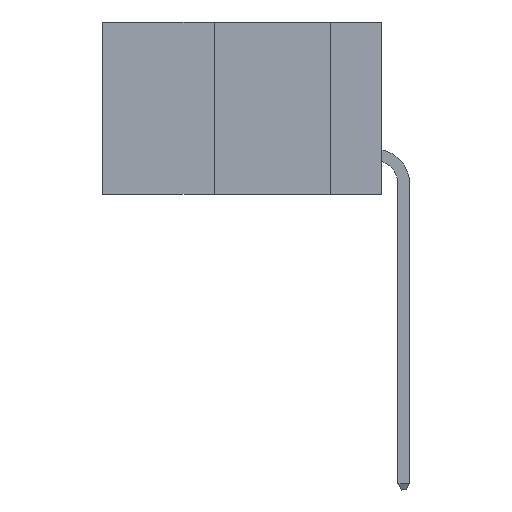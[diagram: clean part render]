
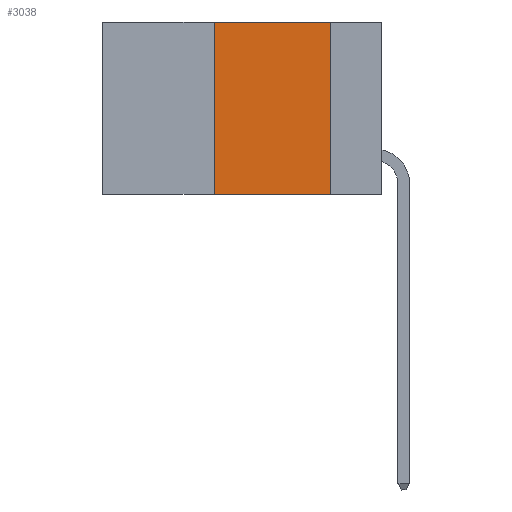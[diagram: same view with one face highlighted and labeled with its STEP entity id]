
A CAD part, left-side view. The second image highlights one B-rep face of the part: STEP entity #3038.
In plain terms, the highlighted planar face has unit normal (-1, 0, 0).
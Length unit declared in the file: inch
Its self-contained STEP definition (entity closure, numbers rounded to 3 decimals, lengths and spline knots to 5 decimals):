
#28 = CARTESIAN_POINT ( 'NONE',  ( 0., 0.36, -0.37 ) ) ;
#169 = DIRECTION ( 'NONE',  ( 0., -1., 0. ) ) ;
#285 = ORIENTED_EDGE ( 'NONE', *, *, #8135, .F. ) ;
#476 = VERTEX_POINT ( 'NONE', #6711 ) ;
#570 = DIRECTION ( 'NONE',  ( 1., 0., 0. ) ) ;
#1291 = ORIENTED_EDGE ( 'NONE', *, *, #11088, .F. ) ;
#1450 = EDGE_LOOP ( 'NONE', ( #8328, #1291, #285, #11662 ) ) ;
#1872 = LINE ( 'NONE', #11894, #10396 ) ;
#3038 = ADVANCED_FACE ( 'NONE', ( #11438 ), #11266, .F. ) ;
#4275 = VERTEX_POINT ( 'NONE', #7048 ) ;
#5135 = VERTEX_POINT ( 'NONE', #7975 ) ;
#5703 = CARTESIAN_POINT ( 'NONE',  ( 0., 0.6, 0. ) ) ;
#5816 = CARTESIAN_POINT ( 'NONE',  ( 0., 0.11, 0. ) ) ;
#6197 = LINE ( 'NONE', #13666, #11407 ) ;
#6268 = VECTOR ( 'NONE', #13114, 39.37008 ) ;
#6703 = DIRECTION ( 'NONE',  ( 0., 0., 1. ) ) ;
#6711 = CARTESIAN_POINT ( 'NONE',  ( 0., 0.36, 0. ) ) ;
#6721 = EDGE_CURVE ( 'NONE', #10384, #4275, #6197, .T. ) ;
#6883 = AXIS2_PLACEMENT_3D ( 'NONE', #7125, #570, #8186 ) ;
#7048 = CARTESIAN_POINT ( 'NONE',  ( 0., 0.11, -0.37 ) ) ;
#7125 = CARTESIAN_POINT ( 'NONE',  ( 0., 0.6, 0. ) ) ;
#7920 = VECTOR ( 'NONE', #169, 39.37008 ) ;
#7975 = CARTESIAN_POINT ( 'NONE',  ( 0., 0.11, 0. ) ) ;
#8135 = EDGE_CURVE ( 'NONE', #10384, #476, #1872, .T. ) ;
#8186 = DIRECTION ( 'NONE',  ( 0., 0., -1. ) ) ;
#8328 = ORIENTED_EDGE ( 'NONE', *, *, #12316, .F. ) ;
#9057 = LINE ( 'NONE', #5816, #6268 ) ;
#10384 = VERTEX_POINT ( 'NONE', #28 ) ;
#10396 = VECTOR ( 'NONE', #6703, 39.37008 ) ;
#11088 = EDGE_CURVE ( 'NONE', #476, #5135, #13454, .T. ) ;
#11266 = PLANE ( 'NONE',  #6883 ) ;
#11407 = VECTOR ( 'NONE', #11566, 39.37008 ) ;
#11438 = FACE_OUTER_BOUND ( 'NONE', #1450, .T. ) ;
#11566 = DIRECTION ( 'NONE',  ( 0., -1., 0. ) ) ;
#11662 = ORIENTED_EDGE ( 'NONE', *, *, #6721, .T. ) ;
#11894 = CARTESIAN_POINT ( 'NONE',  ( 0., 0.36, 0. ) ) ;
#12316 = EDGE_CURVE ( 'NONE', #5135, #4275, #9057, .T. ) ;
#13114 = DIRECTION ( 'NONE',  ( 0., 0., -1. ) ) ;
#13454 = LINE ( 'NONE', #5703, #7920 ) ;
#13666 = CARTESIAN_POINT ( 'NONE',  ( 0., 0.6, -0.37 ) ) ;
